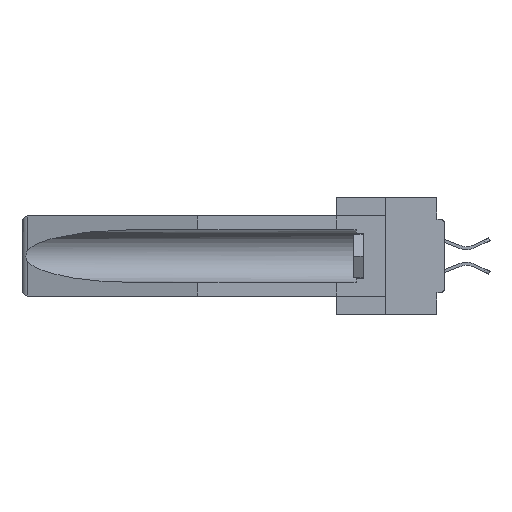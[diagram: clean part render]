
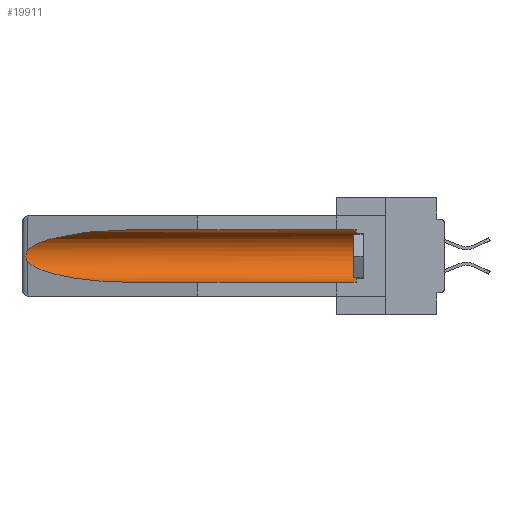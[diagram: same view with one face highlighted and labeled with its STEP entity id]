
A CAD part, left-side view. The second image highlights one B-rep face of the part: STEP entity #19911.
In plain terms, the highlighted cylindrical face has radius 2.857 mm (diameter 5.715 mm), a partial arc.
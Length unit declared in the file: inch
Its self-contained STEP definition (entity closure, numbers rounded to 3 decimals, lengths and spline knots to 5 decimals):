
#367 = ORIENTED_EDGE ( 'NONE', *, *, #41108, .F. ) ;
#3153 = VERTEX_POINT ( 'NONE', #11969 ) ;
#3205 = LINE ( 'NONE', #3968, #15497 ) ;
#3958 = CARTESIAN_POINT ( 'NONE',  ( 0.26537, 1.52718, -0.14972 ) ) ;
#3968 = CARTESIAN_POINT ( 'NONE',  ( 0.155, -0.30754, -0.284 ) ) ;
#4046 = CARTESIAN_POINT ( 'NONE',  ( 0.26537, 1.52718, -0.14972 ) ) ;
#4491 = CARTESIAN_POINT ( 'NONE',  ( 0.25451, 1.48313, -0.09465 ) ) ;
#4902 = ORIENTED_EDGE ( 'NONE', *, *, #29727, .T. ) ;
#5417 = EDGE_CURVE ( 'NONE', #27832, #3153, #23601, .T. ) ;
#7462 = EDGE_CURVE ( 'NONE', #18477, #36748, #34854, .T. ) ;
#9767 = CARTESIAN_POINT ( 'NONE',  ( 0.26537, 1.52718, -0.19328 ) ) ;
#10390 = CARTESIAN_POINT ( 'NONE',  ( 0.155, 1.07973, -0.059 ) ) ;
#10406 = LINE ( 'NONE', #23911, #17348 ) ;
#11969 = CARTESIAN_POINT ( 'NONE',  ( 0.155, 0.126, -0.059 ) ) ;
#12377 =( BOUNDED_CURVE ( )  B_SPLINE_CURVE ( 3, ( #9767, #43916, #35570, #24796 ),
 .UNSPECIFIED., .F., .F. ) 
 B_SPLINE_CURVE_WITH_KNOTS ( ( 4, 4 ),
 ( 0.1948, 1.5708 ),
 .UNSPECIFIED. ) 
 CURVE ( )  GEOMETRIC_REPRESENTATION_ITEM ( )  RATIONAL_B_SPLINE_CURVE ( ( 1., 0.848, 0.848, 1. ) ) 
 REPRESENTATION_ITEM ( '' )  );
#12689 = CARTESIAN_POINT ( 'NONE',  ( 0.155, 1.07973, -0.284 ) ) ;
#14252 = CARTESIAN_POINT ( 'NONE',  ( 0.2673, 1.5327, -0.16383 ) ) ;
#14413 = DIRECTION ( 'NONE',  ( 0., 1., 0. ) ) ;
#14950 = CARTESIAN_POINT ( 'NONE',  ( 0.26537, 1.52718, -0.19328 ) ) ;
#14964 = CARTESIAN_POINT ( 'NONE',  ( 0.26537, 1.52718, -0.14972 ) ) ;
#15497 = VECTOR ( 'NONE', #14413, 39.37008 ) ;
#16204 =( BOUNDED_CURVE ( )  B_SPLINE_CURVE ( 3, ( #28830, #32244, #4491, #14964 ),
 .UNSPECIFIED., .F., .F. ) 
 B_SPLINE_CURVE_WITH_KNOTS ( ( 4, 4 ),
 ( 4.71239, 6.08839 ),
 .UNSPECIFIED. ) 
 CURVE ( )  GEOMETRIC_REPRESENTATION_ITEM ( )  RATIONAL_B_SPLINE_CURVE ( ( 1., 0.848, 0.848, 1. ) ) 
 REPRESENTATION_ITEM ( '' )  );
#16434 = ORIENTED_EDGE ( 'NONE', *, *, #17459, .T. ) ;
#17348 = VECTOR ( 'NONE', #37467, 39.37008 ) ;
#17459 = EDGE_CURVE ( 'NONE', #22787, #18477, #16204, .T. ) ;
#17713 = CARTESIAN_POINT ( 'NONE',  ( 0.2673, 1.53269, -0.17917 ) ) ;
#18180 = DIRECTION ( 'NONE',  ( 0., 1., 0. ) ) ;
#18447 = CARTESIAN_POINT ( 'NONE',  ( 0.26537, 1.52718, -0.19328 ) ) ;
#18477 = VERTEX_POINT ( 'NONE', #4046 ) ;
#19911 = ADVANCED_FACE ( 'NONE', ( #42946 ), #32797, .F. ) ;
#21283 = CARTESIAN_POINT ( 'NONE',  ( 0.26655, 1.53094, -0.18657 ) ) ;
#22787 = VERTEX_POINT ( 'NONE', #10390 ) ;
#23601 = CIRCLE ( 'NONE', #25810, 0.1125 ) ;
#23911 = CARTESIAN_POINT ( 'NONE',  ( 0.155, -0.30754, -0.059 ) ) ;
#24353 = DIRECTION ( 'NONE',  ( 0., 0., 1. ) ) ;
#24545 = VERTEX_POINT ( 'NONE', #12689 ) ;
#24604 = CARTESIAN_POINT ( 'NONE',  ( 0.155, 0.126, -0.284 ) ) ;
#24733 = CARTESIAN_POINT ( 'NONE',  ( 0.26597, 1.5296, -0.19026 ) ) ;
#24796 = CARTESIAN_POINT ( 'NONE',  ( 0.155, 1.07973, -0.284 ) ) ;
#25810 = AXIS2_PLACEMENT_3D ( 'NONE', #34638, #27617, #24353 ) ;
#27617 = DIRECTION ( 'NONE',  ( 0., -1., 0. ) ) ;
#27832 = VERTEX_POINT ( 'NONE', #24604 ) ;
#27846 = CARTESIAN_POINT ( 'NONE',  ( 0.26597, 1.52961, -0.15275 ) ) ;
#28182 = ORIENTED_EDGE ( 'NONE', *, *, #7462, .T. ) ;
#28830 = CARTESIAN_POINT ( 'NONE',  ( 0.155, 1.07973, -0.059 ) ) ;
#29727 = EDGE_CURVE ( 'NONE', #36748, #24545, #12377, .T. ) ;
#29989 = EDGE_LOOP ( 'NONE', ( #16434, #28182, #4902, #367, #36787, #43595 ) ) ;
#32244 = CARTESIAN_POINT ( 'NONE',  ( 0.21114, 1.30732, -0.059 ) ) ;
#32797 = CYLINDRICAL_SURFACE ( 'NONE', #35965, 0.1125 ) ;
#34638 = CARTESIAN_POINT ( 'NONE',  ( 0.155, 0.126, -0.1715 ) ) ;
#34715 = CARTESIAN_POINT ( 'NONE',  ( 0.26654, 1.53092, -0.15636 ) ) ;
#34854 = B_SPLINE_CURVE_WITH_KNOTS ( 'NONE', 3,
 ( #3958, #27846, #34715, #14252, #41678, #35021, #17713, #21283, #24733, #18447 ),
 .UNSPECIFIED., .F., .F.,
 ( 4, 2, 2, 2, 4 ),
 ( 0., 0.00029, 0.00058, 0.00087, 0.00117 ),
 .UNSPECIFIED. ) ;
#35021 = CARTESIAN_POINT ( 'NONE',  ( 0.2675, 1.53308, -0.17534 ) ) ;
#35190 = CARTESIAN_POINT ( 'NONE',  ( 0.155, -0.30754, -0.1715 ) ) ;
#35570 = CARTESIAN_POINT ( 'NONE',  ( 0.21114, 1.30732, -0.284 ) ) ;
#35965 = AXIS2_PLACEMENT_3D ( 'NONE', #35190, #18180, #39050 ) ;
#36748 = VERTEX_POINT ( 'NONE', #14950 ) ;
#36787 = ORIENTED_EDGE ( 'NONE', *, *, #5417, .T. ) ;
#37061 = EDGE_CURVE ( 'NONE', #3153, #22787, #10406, .T. ) ;
#37467 = DIRECTION ( 'NONE',  ( 0., 1., 0. ) ) ;
#39050 = DIRECTION ( 'NONE',  ( 0., 0., 1. ) ) ;
#41108 = EDGE_CURVE ( 'NONE', #27832, #24545, #3205, .T. ) ;
#41678 = CARTESIAN_POINT ( 'NONE',  ( 0.2675, 1.53308, -0.16763 ) ) ;
#42946 = FACE_OUTER_BOUND ( 'NONE', #29989, .T. ) ;
#43595 = ORIENTED_EDGE ( 'NONE', *, *, #37061, .T. ) ;
#43916 = CARTESIAN_POINT ( 'NONE',  ( 0.25451, 1.48313, -0.24835 ) ) ;
